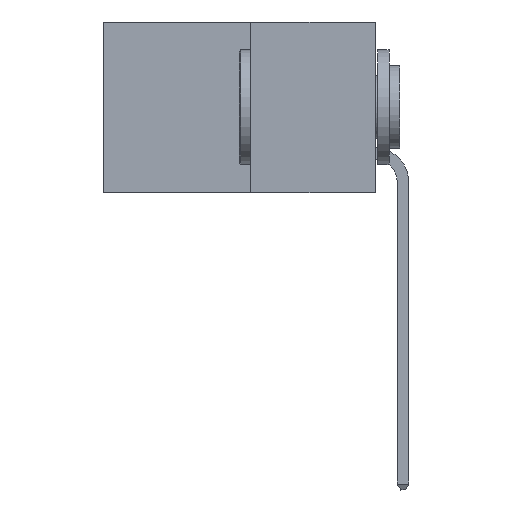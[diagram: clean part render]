
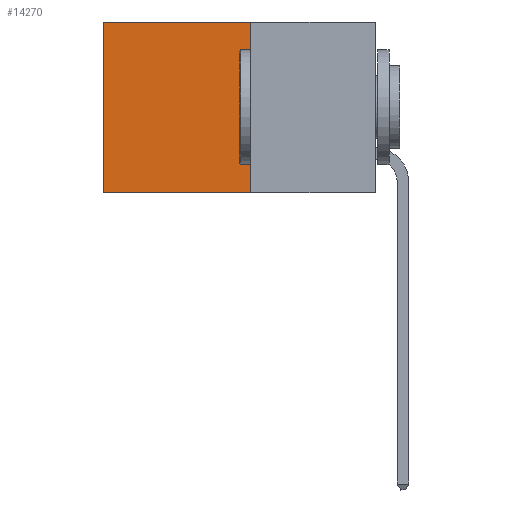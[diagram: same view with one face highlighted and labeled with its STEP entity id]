
A CAD part, left-side view. The second image highlights one B-rep face of the part: STEP entity #14270.
In plain terms, the highlighted planar face has unit normal (-1, 0, 0).
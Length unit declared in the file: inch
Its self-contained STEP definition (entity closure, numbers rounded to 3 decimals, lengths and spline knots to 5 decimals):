
#1055 = DIRECTION ( 'NONE',  ( 1., 0., 0. ) ) ;
#2411 = FACE_OUTER_BOUND ( 'NONE', #2623, .T. ) ;
#2623 = EDGE_LOOP ( 'NONE', ( #11786, #10401, #15089, #14956 ) ) ;
#3389 = EDGE_CURVE ( 'NONE', #9648, #14428, #14268, .T. ) ;
#4670 = AXIS2_PLACEMENT_3D ( 'NONE', #18174, #1055, #11201 ) ;
#4864 = LINE ( 'NONE', #13473, #8249 ) ;
#5777 = CARTESIAN_POINT ( 'NONE',  ( 0.277, 0.27, -0.37 ) ) ;
#5919 = CARTESIAN_POINT ( 'NONE',  ( 0.277, 0.27, 0. ) ) ;
#6244 = CARTESIAN_POINT ( 'NONE',  ( 0.277, 0.27, -0.37 ) ) ;
#6643 = VECTOR ( 'NONE', #11643, 39.37008 ) ;
#6928 = VECTOR ( 'NONE', #13896, 39.37008 ) ;
#7283 = VERTEX_POINT ( 'NONE', #13450 ) ;
#8249 = VECTOR ( 'NONE', #9222, 39.37008 ) ;
#8712 = EDGE_CURVE ( 'NONE', #8907, #7283, #10792, .T. ) ;
#8907 = VERTEX_POINT ( 'NONE', #11433 ) ;
#9222 = DIRECTION ( 'NONE',  ( 0., 1., 0. ) ) ;
#9648 = VERTEX_POINT ( 'NONE', #5919 ) ;
#10401 = ORIENTED_EDGE ( 'NONE', *, *, #13977, .F. ) ;
#10585 = DIRECTION ( 'NONE',  ( 0., 1., 0. ) ) ;
#10649 = EDGE_CURVE ( 'NONE', #9648, #8907, #4864, .T. ) ;
#10792 = LINE ( 'NONE', #18047, #6928 ) ;
#10813 = VECTOR ( 'NONE', #10585, 39.37008 ) ;
#11201 = DIRECTION ( 'NONE',  ( 0., 0., -1. ) ) ;
#11433 = CARTESIAN_POINT ( 'NONE',  ( 0.277, 0.59, 0. ) ) ;
#11619 = CARTESIAN_POINT ( 'NONE',  ( 0.277, 0.27, -0.37 ) ) ;
#11643 = DIRECTION ( 'NONE',  ( 0., 0., -1. ) ) ;
#11786 = ORIENTED_EDGE ( 'NONE', *, *, #8712, .T. ) ;
#13450 = CARTESIAN_POINT ( 'NONE',  ( 0.277, 0.59, -0.37 ) ) ;
#13473 = CARTESIAN_POINT ( 'NONE',  ( 0.277, 0.27, 0. ) ) ;
#13896 = DIRECTION ( 'NONE',  ( 0., 0., -1. ) ) ;
#13977 = EDGE_CURVE ( 'NONE', #14428, #7283, #14565, .T. ) ;
#14268 = LINE ( 'NONE', #11619, #6643 ) ;
#14270 = ADVANCED_FACE ( 'NONE', ( #2411 ), #15410, .F. ) ;
#14428 = VERTEX_POINT ( 'NONE', #5777 ) ;
#14565 = LINE ( 'NONE', #6244, #10813 ) ;
#14956 = ORIENTED_EDGE ( 'NONE', *, *, #10649, .T. ) ;
#15089 = ORIENTED_EDGE ( 'NONE', *, *, #3389, .F. ) ;
#15410 = PLANE ( 'NONE',  #4670 ) ;
#18047 = CARTESIAN_POINT ( 'NONE',  ( 0.277, 0.59, -0.37 ) ) ;
#18174 = CARTESIAN_POINT ( 'NONE',  ( 0.277, 0.27, -0.37 ) ) ;
